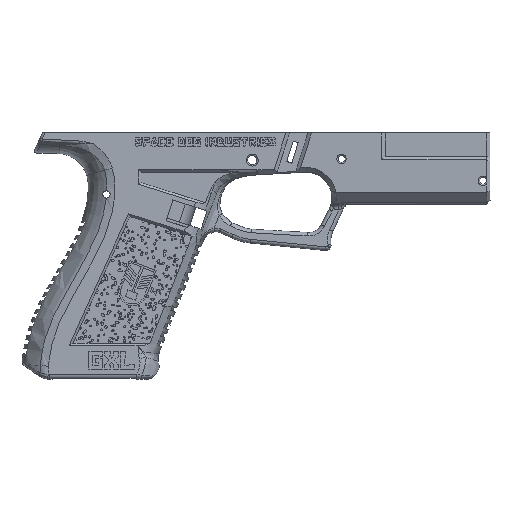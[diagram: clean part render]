
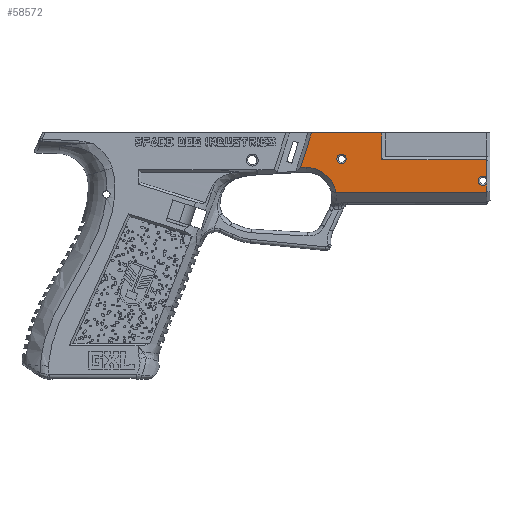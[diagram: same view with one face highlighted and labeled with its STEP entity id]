
A CAD part, top view. The second image highlights one B-rep face of the part: STEP entity #58572.
In plain terms, the highlighted planar face has unit normal (0, 0, 1).
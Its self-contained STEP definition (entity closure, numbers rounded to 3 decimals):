
#2453=FACE_BOUND('',#12777,.T.);
#8100=PLANE('',#62152);
#9197=FACE_OUTER_BOUND('',#12776,.T.);
#12776=EDGE_LOOP('',(#40432,#40433,#40434,#40435,#40436,#40437,#40438,#40439,
#40440,#40441,#40442));
#12777=EDGE_LOOP('',(#40443));
#16940=LINE('',#73505,#20754);
#16941=LINE('',#73507,#20755);
#16942=LINE('',#73509,#20756);
#16943=LINE('',#73511,#20757);
#16944=LINE('',#73513,#20758);
#16945=LINE('',#73515,#20759);
#16946=LINE('',#73519,#20760);
#16947=LINE('',#73520,#20761);
#20754=VECTOR('',#63757,10.);
#20755=VECTOR('',#63758,10.);
#20756=VECTOR('',#63759,10.);
#20757=VECTOR('',#63760,10.);
#20758=VECTOR('',#63761,10.);
#20759=VECTOR('',#63762,10.);
#20760=VECTOR('',#63765,10.);
#20761=VECTOR('',#63766,10.);
#24394=CIRCLE('',#62150,2.);
#24395=CIRCLE('',#62151,2.);
#24396=CIRCLE('',#62153,13.);
#24397=CIRCLE('',#62154,2.025);
#24973=VERTEX_POINT('',#73483);
#24974=VERTEX_POINT('',#73485);
#24975=VERTEX_POINT('',#73487);
#24976=VERTEX_POINT('',#73504);
#24977=VERTEX_POINT('',#73506);
#24978=VERTEX_POINT('',#73508);
#24979=VERTEX_POINT('',#73510);
#24980=VERTEX_POINT('',#73512);
#24981=VERTEX_POINT('',#73514);
#24982=VERTEX_POINT('',#73516);
#24983=VERTEX_POINT('',#73518);
#24984=VERTEX_POINT('',#73521);
#31118=EDGE_CURVE('',#24973,#24974,#24394,.T.);
#31120=EDGE_CURVE('',#24975,#24973,#24395,.T.);
#31121=EDGE_CURVE('',#24976,#24975,#16940,.T.);
#31122=EDGE_CURVE('',#24976,#24977,#16941,.T.);
#31123=EDGE_CURVE('',#24978,#24977,#16942,.T.);
#31124=EDGE_CURVE('',#24979,#24978,#16943,.T.);
#31125=EDGE_CURVE('',#24980,#24979,#16944,.T.);
#31126=EDGE_CURVE('',#24981,#24980,#16945,.T.);
#31127=EDGE_CURVE('',#24982,#24981,#24396,.T.);
#31128=EDGE_CURVE('',#24983,#24982,#16946,.T.);
#31129=EDGE_CURVE('',#24974,#24983,#16947,.T.);
#31130=EDGE_CURVE('',#24984,#24984,#24397,.T.);
#40432=ORIENTED_EDGE('',*,*,#31120,.F.);
#40433=ORIENTED_EDGE('',*,*,#31121,.F.);
#40434=ORIENTED_EDGE('',*,*,#31122,.T.);
#40435=ORIENTED_EDGE('',*,*,#31123,.F.);
#40436=ORIENTED_EDGE('',*,*,#31124,.F.);
#40437=ORIENTED_EDGE('',*,*,#31125,.F.);
#40438=ORIENTED_EDGE('',*,*,#31126,.F.);
#40439=ORIENTED_EDGE('',*,*,#31127,.F.);
#40440=ORIENTED_EDGE('',*,*,#31128,.F.);
#40441=ORIENTED_EDGE('',*,*,#31129,.F.);
#40442=ORIENTED_EDGE('',*,*,#31118,.F.);
#40443=ORIENTED_EDGE('',*,*,#31130,.T.);
#58572=ADVANCED_FACE('',(#9197,#2453),#8100,.F.);
#62150=AXIS2_PLACEMENT_3D('',#73486,#63751,#63752);
#62151=AXIS2_PLACEMENT_3D('',#73502,#63753,#63754);
#62152=AXIS2_PLACEMENT_3D('',#73503,#63755,#63756);
#62153=AXIS2_PLACEMENT_3D('',#73517,#63763,#63764);
#62154=AXIS2_PLACEMENT_3D('',#73522,#63767,#63768);
#63751=DIRECTION('center_axis',(0.,0.,
1.));
#63752=DIRECTION('ref_axis',(-1.,0.,0.));
#63753=DIRECTION('center_axis',(0.,0.,
1.));
#63754=DIRECTION('ref_axis',(-1.,0.,0.));
#63755=DIRECTION('center_axis',(0.,0.,
-1.));
#63756=DIRECTION('ref_axis',(0.,1.,0.));
#63757=DIRECTION('',(0.,-1.,0.));
#63758=DIRECTION('',(-1.,0.,0.));
#63759=DIRECTION('',(0.,-1.,0.));
#63760=DIRECTION('',(1.,0.,0.));
#63761=DIRECTION('',(0.301,0.954,0.));
#63762=DIRECTION('',(-0.999,-0.055,0.));
#63763=DIRECTION('center_axis',(0.,0.,
1.));
#63764=DIRECTION('ref_axis',(0.892,-0.452,0.));
#63765=DIRECTION('',(-1.,0.,0.));
#63766=DIRECTION('',(0.,-1.,0.));
#63767=DIRECTION('center_axis',(0.,0.,
-1.));
#63768=DIRECTION('ref_axis',(0.776,-0.63,0.));
#73483=CARTESIAN_POINT('',(154.135,-18.787,23.145));
#73485=CARTESIAN_POINT('',(157.635,-20.11,23.145));
#73486=CARTESIAN_POINT('Origin',(156.135,-18.787,23.145));
#73487=CARTESIAN_POINT('',(157.635,-17.464,23.145));
#73502=CARTESIAN_POINT('Origin',(156.135,-18.787,23.145));
#73503=CARTESIAN_POINT('Origin',(103.31,1.259,23.145));
#73504=CARTESIAN_POINT('',(157.635,-9.733,23.145));
#73505=CARTESIAN_POINT('',(157.635,-25.087,23.145));
#73506=CARTESIAN_POINT('',(112.635,-9.733,23.145));
#73507=CARTESIAN_POINT('',(105.549,-9.733,23.145));
#73508=CARTESIAN_POINT('',(112.635,1.767,23.145));
#73509=CARTESIAN_POINT('',(112.635,1.513,23.145));
#73510=CARTESIAN_POINT('',(82.591,1.767,23.145));
#73511=CARTESIAN_POINT('',(33.317,1.767,23.145));
#73512=CARTESIAN_POINT('',(77.883,-13.165,23.145));
#73513=CARTESIAN_POINT('',(82.185,0.48,23.145));
#73514=CARTESIAN_POINT('',(80.217,-13.037,23.145));
#73515=CARTESIAN_POINT('',(81.633,-12.959,23.145));
#73516=CARTESIAN_POINT('',(93.078,-23.787,23.145));
#73517=CARTESIAN_POINT('Origin',(80.274,-26.037,23.145));
#73518=CARTESIAN_POINT('',(157.635,-23.787,23.145));
#73519=CARTESIAN_POINT('',(89.618,-23.787,23.145));
#73520=CARTESIAN_POINT('',(157.635,-25.087,23.145));
#73521=CARTESIAN_POINT('',(97.469,-9.398,23.145));
#73522=CARTESIAN_POINT('Origin',(95.444,-9.398,23.145));
